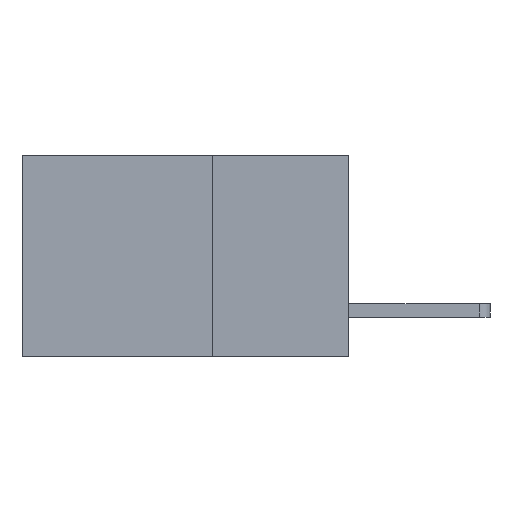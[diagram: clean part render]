
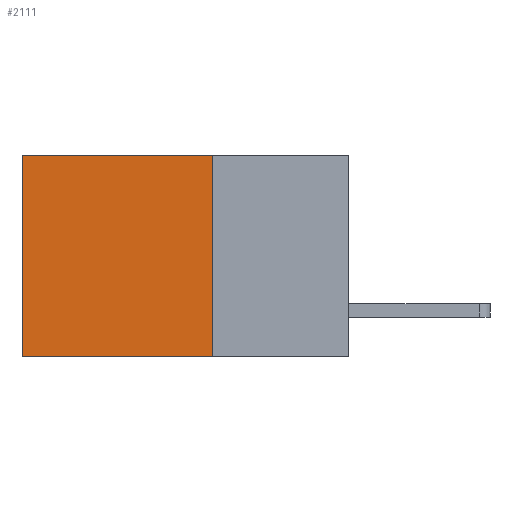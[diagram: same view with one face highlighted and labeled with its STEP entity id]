
A CAD part, left-side view. The second image highlights one B-rep face of the part: STEP entity #2111.
In plain terms, the highlighted planar face has unit normal (-1, 0, 0).
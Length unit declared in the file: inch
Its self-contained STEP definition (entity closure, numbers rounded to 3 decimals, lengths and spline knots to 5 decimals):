
#55 = VERTEX_POINT ( 'NONE', #2171 ) ;
#184 = CARTESIAN_POINT ( 'NONE',  ( 0.2615, 0.25, 0. ) ) ;
#212 = VERTEX_POINT ( 'NONE', #5937 ) ;
#214 = DIRECTION ( 'NONE',  ( 0., 1., 0. ) ) ;
#247 = VERTEX_POINT ( 'NONE', #5631 ) ;
#439 = VECTOR ( 'NONE', #1222, 39.37008 ) ;
#579 = CARTESIAN_POINT ( 'NONE',  ( 0.2615, 0.25, -0.37 ) ) ;
#644 = DIRECTION ( 'NONE',  ( 0., 0., -1. ) ) ;
#1222 = DIRECTION ( 'NONE',  ( 0., 0., -1. ) ) ;
#1693 = EDGE_CURVE ( 'NONE', #212, #55, #7957, .T. ) ;
#1791 = EDGE_LOOP ( 'NONE', ( #6866, #5049, #5829, #6322 ) ) ;
#1893 = CARTESIAN_POINT ( 'NONE',  ( 0.2615, 0.25, -0.37 ) ) ;
#1958 = EDGE_CURVE ( 'NONE', #55, #5989, #2551, .T. ) ;
#2111 = ADVANCED_FACE ( 'NONE', ( #3056 ), #2536, .F. ) ;
#2171 = CARTESIAN_POINT ( 'NONE',  ( 0.2615, 0.6, 0. ) ) ;
#2536 = PLANE ( 'NONE',  #3918 ) ;
#2551 = LINE ( 'NONE', #6171, #5965 ) ;
#2727 = EDGE_CURVE ( 'NONE', #212, #247, #5525, .T. ) ;
#2867 = VECTOR ( 'NONE', #214, 39.37008 ) ;
#3056 = FACE_OUTER_BOUND ( 'NONE', #1791, .T. ) ;
#3248 = CARTESIAN_POINT ( 'NONE',  ( 0.2615, 0.6, -0.37 ) ) ;
#3918 = AXIS2_PLACEMENT_3D ( 'NONE', #1893, #4468, #644 ) ;
#4148 = VECTOR ( 'NONE', #7163, 39.37008 ) ;
#4468 = DIRECTION ( 'NONE',  ( 1., 0., 0. ) ) ;
#5049 = ORIENTED_EDGE ( 'NONE', *, *, #6757, .F. ) ;
#5235 = CARTESIAN_POINT ( 'NONE',  ( 0.2615, 0.25, -0.37 ) ) ;
#5525 = LINE ( 'NONE', #579, #439 ) ;
#5631 = CARTESIAN_POINT ( 'NONE',  ( 0.2615, 0.25, -0.37 ) ) ;
#5829 = ORIENTED_EDGE ( 'NONE', *, *, #2727, .F. ) ;
#5845 = LINE ( 'NONE', #5235, #4148 ) ;
#5937 = CARTESIAN_POINT ( 'NONE',  ( 0.2615, 0.25, 0. ) ) ;
#5965 = VECTOR ( 'NONE', #8074, 39.37008 ) ;
#5989 = VERTEX_POINT ( 'NONE', #3248 ) ;
#6171 = CARTESIAN_POINT ( 'NONE',  ( 0.2615, 0.6, -0.37 ) ) ;
#6322 = ORIENTED_EDGE ( 'NONE', *, *, #1693, .T. ) ;
#6757 = EDGE_CURVE ( 'NONE', #247, #5989, #5845, .T. ) ;
#6866 = ORIENTED_EDGE ( 'NONE', *, *, #1958, .T. ) ;
#7163 = DIRECTION ( 'NONE',  ( 0., 1., 0. ) ) ;
#7957 = LINE ( 'NONE', #184, #2867 ) ;
#8074 = DIRECTION ( 'NONE',  ( 0., 0., -1. ) ) ;
